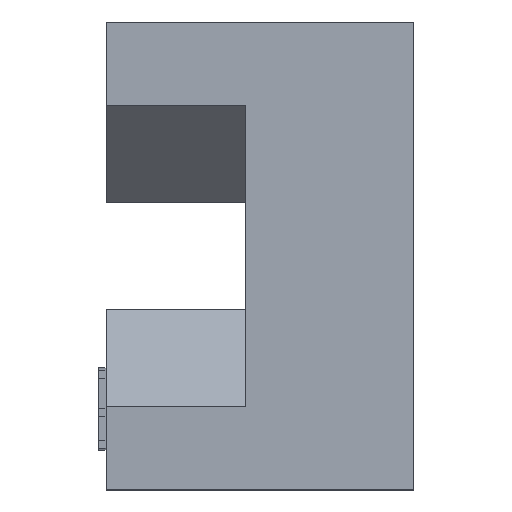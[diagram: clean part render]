
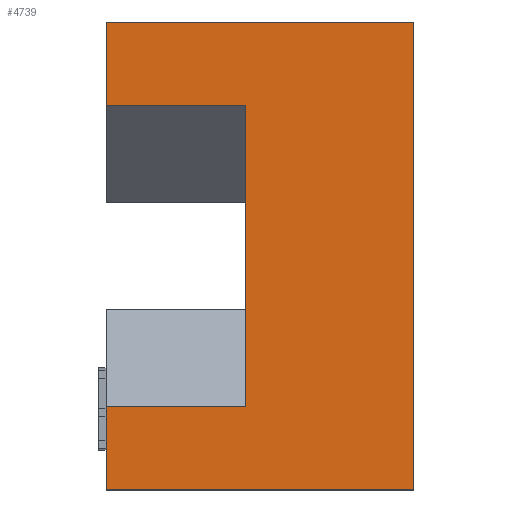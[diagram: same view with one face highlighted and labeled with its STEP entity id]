
A CAD part, left-side view. The second image highlights one B-rep face of the part: STEP entity #4739.
In plain terms, the highlighted planar face has unit normal (-1, 0, 0).
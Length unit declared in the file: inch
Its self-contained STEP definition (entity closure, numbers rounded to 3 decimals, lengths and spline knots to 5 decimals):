
#79 = EDGE_CURVE ( 'NONE', #10611, #12390, #10114, .T. ) ;
#509 = EDGE_CURVE ( 'NONE', #12390, #12808, #7215, .T. ) ;
#730 = CARTESIAN_POINT ( 'NONE',  ( -5.5, 0.205, 0.156 ) ) ;
#936 = CARTESIAN_POINT ( 'NONE',  ( -5.5, 0.112, -0.1005 ) ) ;
#1084 = LINE ( 'NONE', #4109, #13900 ) ;
#1357 = CARTESIAN_POINT ( 'NONE',  ( -5.5, 0.205, -0.156 ) ) ;
#1955 = CARTESIAN_POINT ( 'NONE',  ( -5.5, 0., 0.156 ) ) ;
#2001 = AXIS2_PLACEMENT_3D ( 'NONE', #10788, #7879, #13386 ) ;
#2310 = VECTOR ( 'NONE', #12020, 39.37008 ) ;
#2323 = CARTESIAN_POINT ( 'NONE',  ( -5.5, 0.205, -0.156 ) ) ;
#2362 = CARTESIAN_POINT ( 'NONE',  ( -5.5, 0.112, 0.1005 ) ) ;
#2441 = ORIENTED_EDGE ( 'NONE', *, *, #14511, .F. ) ;
#2585 = VECTOR ( 'NONE', #8737, 39.37008 ) ;
#2935 = LINE ( 'NONE', #4121, #2310 ) ;
#3311 = LINE ( 'NONE', #12241, #4198 ) ;
#3312 = CARTESIAN_POINT ( 'NONE',  ( -5.5, 0.205, -0.1005 ) ) ;
#3317 = LINE ( 'NONE', #6365, #2585 ) ;
#3940 = FACE_OUTER_BOUND ( 'NONE', #11561, .T. ) ;
#4109 = CARTESIAN_POINT ( 'NONE',  ( -5.5, 0.112, -0.1005 ) ) ;
#4121 = CARTESIAN_POINT ( 'NONE',  ( -5.5, 0.205, -0.156 ) ) ;
#4198 = VECTOR ( 'NONE', #4340, 39.37008 ) ;
#4314 = ORIENTED_EDGE ( 'NONE', *, *, #11875, .F. ) ;
#4340 = DIRECTION ( 'NONE',  ( 0., -1., 0. ) ) ;
#4739 = ADVANCED_FACE ( 'NONE', ( #3940 ), #6245, .F. ) ;
#5288 = ORIENTED_EDGE ( 'NONE', *, *, #509, .T. ) ;
#5770 = VECTOR ( 'NONE', #5893, 39.37008 ) ;
#5893 = DIRECTION ( 'NONE',  ( 0., 0., 1. ) ) ;
#6146 = CARTESIAN_POINT ( 'NONE',  ( -5.5, 0.112, -0.1005 ) ) ;
#6245 = PLANE ( 'NONE',  #2001 ) ;
#6267 = EDGE_CURVE ( 'NONE', #8304, #7302, #1084, .T. ) ;
#6365 = CARTESIAN_POINT ( 'NONE',  ( -5.5, 0.205, -0.156 ) ) ;
#6676 = CARTESIAN_POINT ( 'NONE',  ( -5.5, 0.112, 0.1005 ) ) ;
#7139 = ORIENTED_EDGE ( 'NONE', *, *, #79, .T. ) ;
#7215 = LINE ( 'NONE', #9454, #5770 ) ;
#7302 = VERTEX_POINT ( 'NONE', #3312 ) ;
#7356 = ORIENTED_EDGE ( 'NONE', *, *, #12110, .F. ) ;
#7605 = DIRECTION ( 'NONE',  ( 0., 1., 0. ) ) ;
#7812 = DIRECTION ( 'NONE',  ( 0., -1., 0. ) ) ;
#7879 = DIRECTION ( 'NONE',  ( 1., 0., 0. ) ) ;
#8304 = VERTEX_POINT ( 'NONE', #936 ) ;
#8474 = ORIENTED_EDGE ( 'NONE', *, *, #14709, .F. ) ;
#8737 = DIRECTION ( 'NONE',  ( 0., 0., 1. ) ) ;
#8845 = VERTEX_POINT ( 'NONE', #13160 ) ;
#9131 = VERTEX_POINT ( 'NONE', #730 ) ;
#9418 = DIRECTION ( 'NONE',  ( 0., 0., 1. ) ) ;
#9454 = CARTESIAN_POINT ( 'NONE',  ( -5.5, 0., -0.156 ) ) ;
#9629 = CARTESIAN_POINT ( 'NONE',  ( -5.5, 0., -0.156 ) ) ;
#10043 = VERTEX_POINT ( 'NONE', #6676 ) ;
#10046 = ORIENTED_EDGE ( 'NONE', *, *, #12413, .F. ) ;
#10114 = LINE ( 'NONE', #1357, #11704 ) ;
#10310 = DIRECTION ( 'NONE',  ( 0., 1., 0. ) ) ;
#10611 = VERTEX_POINT ( 'NONE', #2323 ) ;
#10788 = CARTESIAN_POINT ( 'NONE',  ( -5.5, 0.205, -0.156 ) ) ;
#11561 = EDGE_LOOP ( 'NONE', ( #2441, #13760, #8474, #7139, #5288, #7356, #10046, #4314 ) ) ;
#11704 = VECTOR ( 'NONE', #7812, 39.37008 ) ;
#11807 = LINE ( 'NONE', #6146, #11853 ) ;
#11853 = VECTOR ( 'NONE', #9418, 39.37008 ) ;
#11875 = EDGE_CURVE ( 'NONE', #10043, #8845, #12481, .T. ) ;
#12020 = DIRECTION ( 'NONE',  ( 0., 0., 1. ) ) ;
#12110 = EDGE_CURVE ( 'NONE', #9131, #12808, #3311, .T. ) ;
#12241 = CARTESIAN_POINT ( 'NONE',  ( -5.5, 0.205, 0.156 ) ) ;
#12294 = VECTOR ( 'NONE', #10310, 39.37008 ) ;
#12390 = VERTEX_POINT ( 'NONE', #9629 ) ;
#12413 = EDGE_CURVE ( 'NONE', #8845, #9131, #2935, .T. ) ;
#12481 = LINE ( 'NONE', #2362, #12294 ) ;
#12808 = VERTEX_POINT ( 'NONE', #1955 ) ;
#13160 = CARTESIAN_POINT ( 'NONE',  ( -5.5, 0.205, 0.1005 ) ) ;
#13386 = DIRECTION ( 'NONE',  ( 0., 0., -1. ) ) ;
#13760 = ORIENTED_EDGE ( 'NONE', *, *, #6267, .T. ) ;
#13900 = VECTOR ( 'NONE', #7605, 39.37008 ) ;
#14511 = EDGE_CURVE ( 'NONE', #8304, #10043, #11807, .T. ) ;
#14709 = EDGE_CURVE ( 'NONE', #10611, #7302, #3317, .T. ) ;
